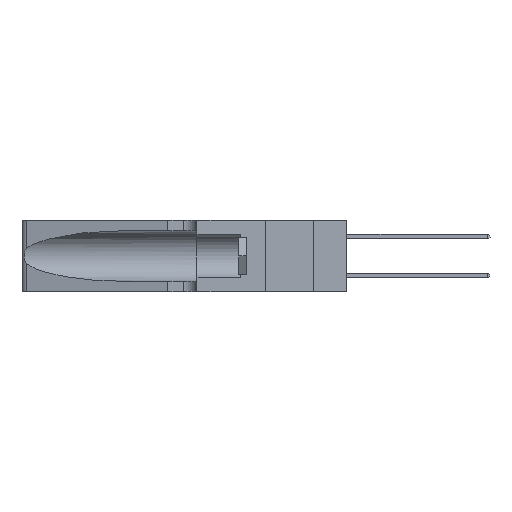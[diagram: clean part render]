
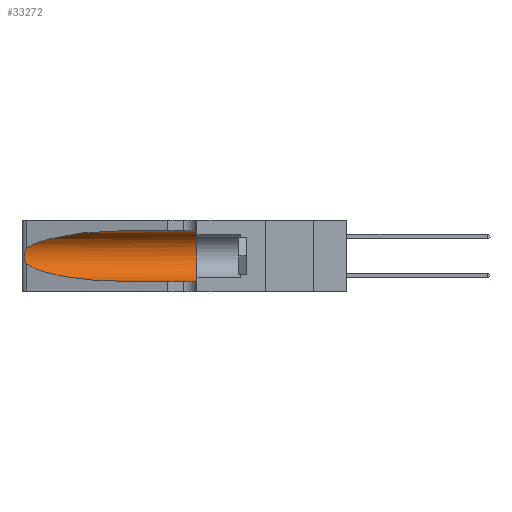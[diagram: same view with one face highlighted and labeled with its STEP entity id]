
A CAD part, left-side view. The second image highlights one B-rep face of the part: STEP entity #33272.
In plain terms, the highlighted cylindrical face has radius 3.308 mm (diameter 6.617 mm), a partial arc.
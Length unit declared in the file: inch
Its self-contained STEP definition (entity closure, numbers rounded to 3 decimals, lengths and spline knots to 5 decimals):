
#172 = CARTESIAN_POINT ( 'NONE',  ( 0.25555, 1.22994, 0.2215 ) ) ;
#2472 = DIRECTION ( 'NONE',  ( 0., 0., 1. ) ) ;
#6096 =( BOUNDED_CURVE ( )  B_SPLINE_CURVE ( 3, ( #8817, #15443, #15021, #21686 ),
 .UNSPECIFIED., .F., .T. ) 
 B_SPLINE_CURVE_WITH_KNOTS ( ( 4, 4 ),
 ( 3.44316, 4.71239 ),
 .UNSPECIFIED. ) 
 CURVE ( )  GEOMETRIC_REPRESENTATION_ITEM ( )  RATIONAL_B_SPLINE_CURVE ( ( 1., 0.87, 0.87, 1. ) ) 
 REPRESENTATION_ITEM ( '' )  );
#6389 = CARTESIAN_POINT ( 'NONE',  ( 0.25487, 1.22718, 0.14631 ) ) ;
#6531 = CARTESIAN_POINT ( 'NONE',  ( 0.25787, 1.23484, 0.2124 ) ) ;
#6683 = CARTESIAN_POINT ( 'NONE',  ( 0.25854, 1.2359, 0.20912 ) ) ;
#6829 = CARTESIAN_POINT ( 'NONE',  ( 0.25487, 1.22718, 0.14631 ) ) ;
#8390 = LINE ( 'NONE', #9472, #41528 ) ;
#8692 = VERTEX_POINT ( 'NONE', #26904 ) ;
#8817 = CARTESIAN_POINT ( 'NONE',  ( 0.25487, 1.22718, 0.14631 ) ) ;
#9472 = CARTESIAN_POINT ( 'NONE',  ( 0.1305, 1.61858, 0.31525 ) ) ;
#9872 = CARTESIAN_POINT ( 'NONE',  ( 0.25789, 1.23486, 0.15765 ) ) ;
#10014 = CARTESIAN_POINT ( 'NONE',  ( 0.26017, 1.23833, 0.17102 ) ) ;
#10397 = VERTEX_POINT ( 'NONE', #33776 ) ;
#12142 = CARTESIAN_POINT ( 'NONE',  ( 0.1305, 0.35, 0.185 ) ) ;
#12289 = DIRECTION ( 'NONE',  ( 0., 1., 0. ) ) ;
#12707 = VECTOR ( 'NONE', #36378, 39.37008 ) ;
#13110 = CARTESIAN_POINT ( 'NONE',  ( 0.1305, 0.72297, 0.05475 ) ) ;
#13344 = CARTESIAN_POINT ( 'NONE',  ( 0.25639, 1.23186, 0.15144 ) ) ;
#13541 = CARTESIAN_POINT ( 'NONE',  ( 0.1305, 1.61858, 0.05475 ) ) ;
#14403 = EDGE_CURVE ( 'NONE', #36855, #41361, #24402, .T. ) ;
#14901 = VERTEX_POINT ( 'NONE', #6829 ) ;
#15021 = CARTESIAN_POINT ( 'NONE',  ( 0.18966, 0.96281, 0.05475 ) ) ;
#15443 = CARTESIAN_POINT ( 'NONE',  ( 0.2373, 1.15595, 0.08982 ) ) ;
#16247 = EDGE_LOOP ( 'NONE', ( #30288, #36497, #30041, #25584, #23085, #35901 ) ) ;
#16719 = B_SPLINE_CURVE_WITH_KNOTS ( 'NONE', 3,
 ( #26348, #172, #23296, #6531, #6683, #42602, #29671, #29809, #10014, #33152, #9872, #13344, #19699, #6389 ),
 .UNSPECIFIED., .F., .F.,
 ( 4, 2, 2, 2, 2, 2, 4 ),
 ( 0., 0.00027, 0.00053, 0.00107, 0.0016, 0.00187, 0.00214 ),
 .UNSPECIFIED. ) ;
#19699 = CARTESIAN_POINT ( 'NONE',  ( 0.25555, 1.22993, 0.14849 ) ) ;
#19862 = CARTESIAN_POINT ( 'NONE',  ( 0.1305, 0.72297, 0.31525 ) ) ;
#21686 = CARTESIAN_POINT ( 'NONE',  ( 0.1305, 0.72297, 0.05475 ) ) ;
#23085 = ORIENTED_EDGE ( 'NONE', *, *, #41481, .F. ) ;
#23296 = CARTESIAN_POINT ( 'NONE',  ( 0.25639, 1.23184, 0.21858 ) ) ;
#24351 = CARTESIAN_POINT ( 'NONE',  ( 0.25487, 1.22718, 0.22369 ) ) ;
#24402 =( BOUNDED_CURVE ( )  B_SPLINE_CURVE ( 3, ( #27533, #40440, #30748, #24351 ),
 .UNSPECIFIED., .F., .T. ) 
 B_SPLINE_CURVE_WITH_KNOTS ( ( 4, 4 ),
 ( 1.5708, 2.84003 ),
 .UNSPECIFIED. ) 
 CURVE ( )  GEOMETRIC_REPRESENTATION_ITEM ( )  RATIONAL_B_SPLINE_CURVE ( ( 1., 0.87, 0.87, 1. ) ) 
 REPRESENTATION_ITEM ( '' )  );
#24872 = CARTESIAN_POINT ( 'NONE',  ( 0.25487, 1.22718, 0.22369 ) ) ;
#25584 = ORIENTED_EDGE ( 'NONE', *, *, #27523, .T. ) ;
#26041 = AXIS2_PLACEMENT_3D ( 'NONE', #31183, #27691, #34241 ) ;
#26287 = EDGE_CURVE ( 'NONE', #41361, #14901, #16719, .T. ) ;
#26348 = CARTESIAN_POINT ( 'NONE',  ( 0.25487, 1.22718, 0.22369 ) ) ;
#26904 = CARTESIAN_POINT ( 'NONE',  ( 0.1305, 0.35, 0.31525 ) ) ;
#27523 = EDGE_CURVE ( 'NONE', #34254, #10397, #30305, .T. ) ;
#27533 = CARTESIAN_POINT ( 'NONE',  ( 0.1305, 0.72297, 0.31525 ) ) ;
#27691 = DIRECTION ( 'NONE',  ( 0., -1., 0. ) ) ;
#29671 = CARTESIAN_POINT ( 'NONE',  ( 0.26075, 1.23896, 0.19203 ) ) ;
#29809 = CARTESIAN_POINT ( 'NONE',  ( 0.26075, 1.23896, 0.178 ) ) ;
#29884 = AXIS2_PLACEMENT_3D ( 'NONE', #12142, #12289, #2472 ) ;
#30041 = ORIENTED_EDGE ( 'NONE', *, *, #39340, .T. ) ;
#30288 = ORIENTED_EDGE ( 'NONE', *, *, #14403, .T. ) ;
#30305 = LINE ( 'NONE', #13541, #12707 ) ;
#30748 = CARTESIAN_POINT ( 'NONE',  ( 0.2373, 1.15595, 0.28018 ) ) ;
#31183 = CARTESIAN_POINT ( 'NONE',  ( 0.1305, 1.61858, 0.185 ) ) ;
#33152 = CARTESIAN_POINT ( 'NONE',  ( 0.25856, 1.23593, 0.16098 ) ) ;
#33272 = ADVANCED_FACE ( 'NONE', ( #33885 ), #38036, .F. ) ;
#33776 = CARTESIAN_POINT ( 'NONE',  ( 0.1305, 0.35, 0.05475 ) ) ;
#33885 = FACE_OUTER_BOUND ( 'NONE', #16247, .T. ) ;
#34241 = DIRECTION ( 'NONE',  ( 0., 0., -1. ) ) ;
#34254 = VERTEX_POINT ( 'NONE', #13110 ) ;
#35176 = CIRCLE ( 'NONE', #29884, 0.13025 ) ;
#35901 = ORIENTED_EDGE ( 'NONE', *, *, #40243, .F. ) ;
#35924 = DIRECTION ( 'NONE',  ( 0., -1., 0. ) ) ;
#36378 = DIRECTION ( 'NONE',  ( 0., -1., 0. ) ) ;
#36497 = ORIENTED_EDGE ( 'NONE', *, *, #26287, .T. ) ;
#36855 = VERTEX_POINT ( 'NONE', #19862 ) ;
#38036 = CYLINDRICAL_SURFACE ( 'NONE', #26041, 0.13025 ) ;
#39340 = EDGE_CURVE ( 'NONE', #14901, #34254, #6096, .T. ) ;
#40243 = EDGE_CURVE ( 'NONE', #36855, #8692, #8390, .T. ) ;
#40440 = CARTESIAN_POINT ( 'NONE',  ( 0.18966, 0.96281, 0.31525 ) ) ;
#41361 = VERTEX_POINT ( 'NONE', #24872 ) ;
#41481 = EDGE_CURVE ( 'NONE', #8692, #10397, #35176, .T. ) ;
#41528 = VECTOR ( 'NONE', #35924, 39.37008 ) ;
#42602 = CARTESIAN_POINT ( 'NONE',  ( 0.26018, 1.23835, 0.19895 ) ) ;
